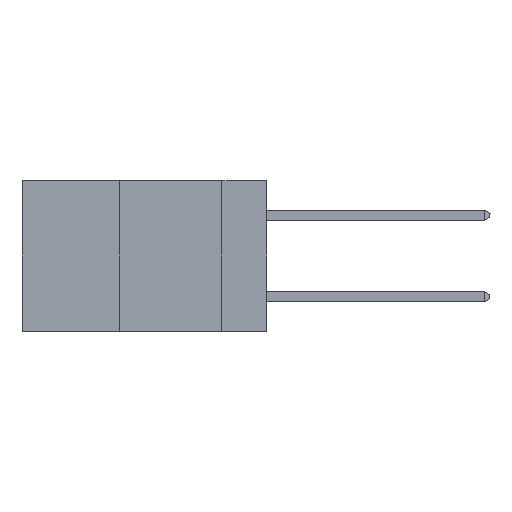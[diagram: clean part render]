
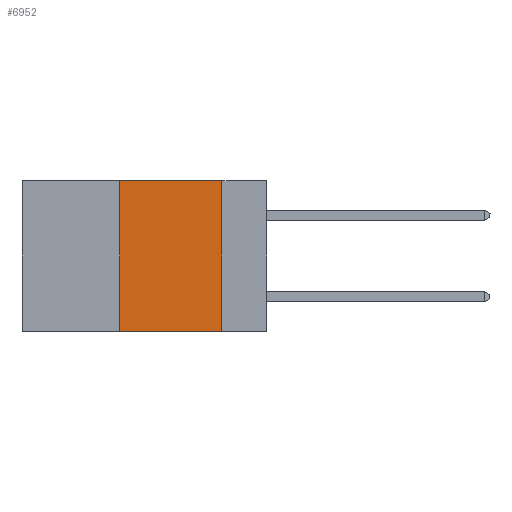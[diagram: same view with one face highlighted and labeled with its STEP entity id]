
A CAD part, left-side view. The second image highlights one B-rep face of the part: STEP entity #6952.
In plain terms, the highlighted planar face has unit normal (-1, 0, 0).
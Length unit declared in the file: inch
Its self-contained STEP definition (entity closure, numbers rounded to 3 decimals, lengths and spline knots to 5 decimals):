
#800 = VECTOR ( 'NONE', #6695, 39.37008 ) ;
#1156 = CARTESIAN_POINT ( 'NONE',  ( 0., 0.36, -0.37 ) ) ;
#1497 = VERTEX_POINT ( 'NONE', #6025 ) ;
#1513 = LINE ( 'NONE', #7673, #5756 ) ;
#1795 = ORIENTED_EDGE ( 'NONE', *, *, #9681, .F. ) ;
#2259 = VECTOR ( 'NONE', #4207, 39.37008 ) ;
#2634 = ORIENTED_EDGE ( 'NONE', *, *, #9084, .T. ) ;
#2813 = CARTESIAN_POINT ( 'NONE',  ( 0., 0.36, 0. ) ) ;
#3370 = CARTESIAN_POINT ( 'NONE',  ( 0., 0.6, -0.37 ) ) ;
#4142 = CARTESIAN_POINT ( 'NONE',  ( 0., 0.6, 0. ) ) ;
#4207 = DIRECTION ( 'NONE',  ( 0., -1., 0. ) ) ;
#4389 = LINE ( 'NONE', #3370, #2259 ) ;
#4895 = DIRECTION ( 'NONE',  ( 1., 0., 0. ) ) ;
#4967 = AXIS2_PLACEMENT_3D ( 'NONE', #11210, #4895, #10233 ) ;
#5015 = LINE ( 'NONE', #4142, #800 ) ;
#5650 = EDGE_LOOP ( 'NONE', ( #11255, #7847, #1795, #2634 ) ) ;
#5704 = PLANE ( 'NONE',  #4967 ) ;
#5756 = VECTOR ( 'NONE', #9686, 39.37008 ) ;
#6025 = CARTESIAN_POINT ( 'NONE',  ( 0., 0.11, -0.37 ) ) ;
#6128 = VERTEX_POINT ( 'NONE', #10015 ) ;
#6429 = VERTEX_POINT ( 'NONE', #2813 ) ;
#6695 = DIRECTION ( 'NONE',  ( 0., -1., 0. ) ) ;
#6793 = CARTESIAN_POINT ( 'NONE',  ( 0., 0.11, 0. ) ) ;
#6952 = ADVANCED_FACE ( 'NONE', ( #8067 ), #5704, .F. ) ;
#7673 = CARTESIAN_POINT ( 'NONE',  ( 0., 0.36, 0. ) ) ;
#7847 = ORIENTED_EDGE ( 'NONE', *, *, #11326, .F. ) ;
#8067 = FACE_OUTER_BOUND ( 'NONE', #5650, .T. ) ;
#9084 = EDGE_CURVE ( 'NONE', #9191, #1497, #4389, .T. ) ;
#9191 = VERTEX_POINT ( 'NONE', #1156 ) ;
#9681 = EDGE_CURVE ( 'NONE', #9191, #6429, #1513, .T. ) ;
#9686 = DIRECTION ( 'NONE',  ( 0., 0., 1. ) ) ;
#10015 = CARTESIAN_POINT ( 'NONE',  ( 0., 0.11, 0. ) ) ;
#10233 = DIRECTION ( 'NONE',  ( 0., 0., -1. ) ) ;
#10243 = LINE ( 'NONE', #6793, #11218 ) ;
#10327 = DIRECTION ( 'NONE',  ( 0., 0., -1. ) ) ;
#10938 = EDGE_CURVE ( 'NONE', #6128, #1497, #10243, .T. ) ;
#11210 = CARTESIAN_POINT ( 'NONE',  ( 0., 0.6, 0. ) ) ;
#11218 = VECTOR ( 'NONE', #10327, 39.37008 ) ;
#11255 = ORIENTED_EDGE ( 'NONE', *, *, #10938, .F. ) ;
#11326 = EDGE_CURVE ( 'NONE', #6429, #6128, #5015, .T. ) ;
